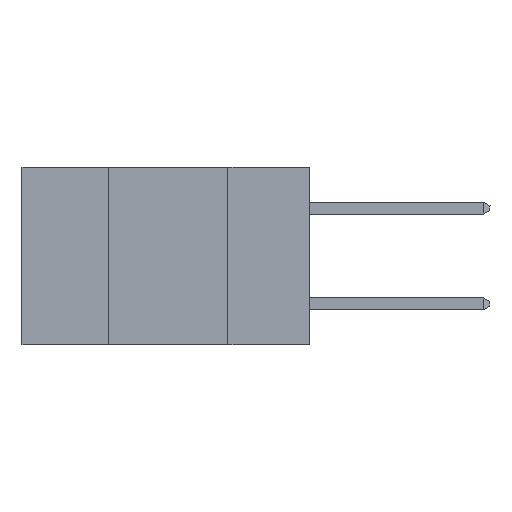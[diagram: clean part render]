
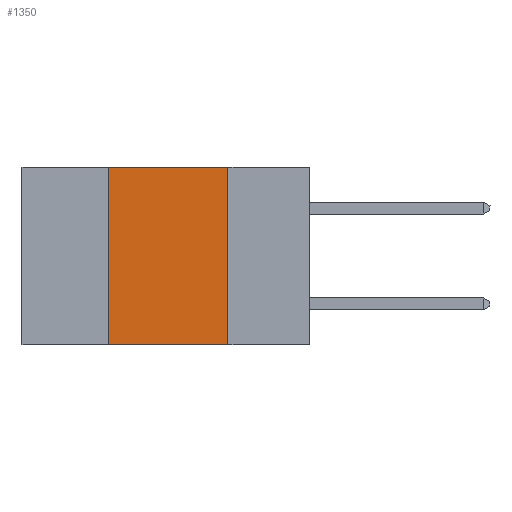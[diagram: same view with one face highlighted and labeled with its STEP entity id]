
A CAD part, left-side view. The second image highlights one B-rep face of the part: STEP entity #1350.
In plain terms, the highlighted planar face has unit normal (-1, 0, 0).
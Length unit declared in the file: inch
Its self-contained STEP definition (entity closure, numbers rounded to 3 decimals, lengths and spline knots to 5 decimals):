
#584 = CARTESIAN_POINT ( 'NONE',  ( 0., 0.42, 0. ) ) ;
#1350 = ADVANCED_FACE ( 'NONE', ( #2314 ), #11318, .F. ) ;
#1484 = CARTESIAN_POINT ( 'NONE',  ( 0., 0.17, 0. ) ) ;
#1720 = VECTOR ( 'NONE', #5867, 39.37008 ) ;
#1752 = AXIS2_PLACEMENT_3D ( 'NONE', #11295, #11218, #11280 ) ;
#1812 = ORIENTED_EDGE ( 'NONE', *, *, #11038, .F. ) ;
#2314 = FACE_OUTER_BOUND ( 'NONE', #13137, .T. ) ;
#2372 = EDGE_CURVE ( 'NONE', #10813, #5233, #7333, .T. ) ;
#2635 = VECTOR ( 'NONE', #7723, 39.37008 ) ;
#3097 = LINE ( 'NONE', #8096, #6638 ) ;
#3518 = DIRECTION ( 'NONE',  ( 0., -1., 0. ) ) ;
#3639 = CARTESIAN_POINT ( 'NONE',  ( 0., 0.6, -0.37 ) ) ;
#5233 = VERTEX_POINT ( 'NONE', #11583 ) ;
#5867 = DIRECTION ( 'NONE',  ( 0., 0., -1. ) ) ;
#6638 = VECTOR ( 'NONE', #15092, 39.37008 ) ;
#7333 = LINE ( 'NONE', #3639, #13089 ) ;
#7723 = DIRECTION ( 'NONE',  ( 0., 0., 1. ) ) ;
#8096 = CARTESIAN_POINT ( 'NONE',  ( 0., 0.6, 0. ) ) ;
#8198 = ORIENTED_EDGE ( 'NONE', *, *, #2372, .T. ) ;
#9624 = EDGE_CURVE ( 'NONE', #12130, #5233, #14295, .T. ) ;
#10042 = CARTESIAN_POINT ( 'NONE',  ( 0., 0.42, 0. ) ) ;
#10187 = ORIENTED_EDGE ( 'NONE', *, *, #9624, .F. ) ;
#10813 = VERTEX_POINT ( 'NONE', #10888 ) ;
#10888 = CARTESIAN_POINT ( 'NONE',  ( 0., 0.42, -0.37 ) ) ;
#11038 = EDGE_CURVE ( 'NONE', #10813, #14941, #14777, .T. ) ;
#11218 = DIRECTION ( 'NONE',  ( 1., 0., 0. ) ) ;
#11280 = DIRECTION ( 'NONE',  ( 0., 0., -1. ) ) ;
#11295 = CARTESIAN_POINT ( 'NONE',  ( 0., 0.6, 0. ) ) ;
#11318 = PLANE ( 'NONE',  #1752 ) ;
#11583 = CARTESIAN_POINT ( 'NONE',  ( 0., 0.17, -0.37 ) ) ;
#12130 = VERTEX_POINT ( 'NONE', #1484 ) ;
#12760 = CARTESIAN_POINT ( 'NONE',  ( 0., 0.17, 0. ) ) ;
#13089 = VECTOR ( 'NONE', #3518, 39.37008 ) ;
#13137 = EDGE_LOOP ( 'NONE', ( #10187, #13601, #1812, #8198 ) ) ;
#13601 = ORIENTED_EDGE ( 'NONE', *, *, #14424, .F. ) ;
#14295 = LINE ( 'NONE', #12760, #1720 ) ;
#14424 = EDGE_CURVE ( 'NONE', #14941, #12130, #3097, .T. ) ;
#14777 = LINE ( 'NONE', #10042, #2635 ) ;
#14941 = VERTEX_POINT ( 'NONE', #584 ) ;
#15092 = DIRECTION ( 'NONE',  ( 0., -1., 0. ) ) ;
